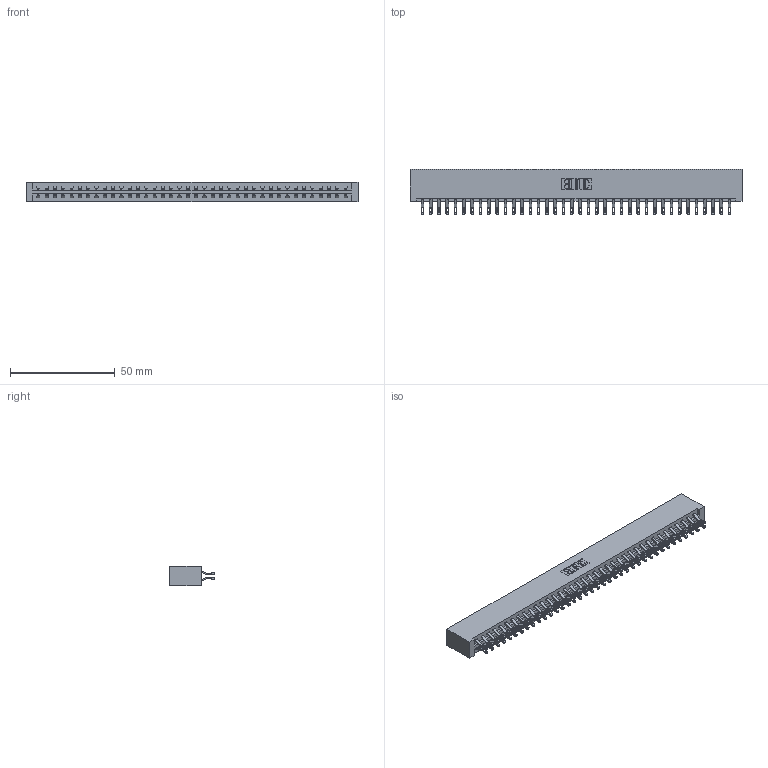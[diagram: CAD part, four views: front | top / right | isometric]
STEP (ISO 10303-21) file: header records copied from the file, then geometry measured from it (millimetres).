
FILE_DESCRIPTION (( 'STEP AP203' ), '1' );
FILE_NAME ('387-076-555-201.STEP', '2018-09-23T15:59:29', ( '' ), ( '' ), 'SwSTEP 2.0', 'SolidWorks 2016', '' );
FILE_SCHEMA (( 'CONFIG_CONTROL_DESIGN' ));
Length unit declared in the file: inch
Products named in the file (3): 337 Part_No Mounting Lugs; 345-292-001_555 Tail; 387-076-555-201
Assembly tree (77 placements, depth 2):
  387-076-555-201
    337 Part_No Mounting Lugs
    345-292-001_555 Tail  x76
Bounding box: 158.45 x 21.47 x 9.4 mm (x, y, z)
Volume: 17626.1 mm3; surface area: 20774.4 mm2
Topology: 77 solids, 77 shells, 4666 faces, 14651 edges, 9766 vertices
Faces by surface type: plane 2802, cylinder 1864
Entity records: 30029 total; most frequent: CARTESIAN_POINT 5096, ORIENTED_EDGE 5002, DIRECTION 4305, EDGE_CURVE 2501, VECTOR 2361, LINE 2361, VERTEX_POINT 1666, AXIS2_PLACEMENT_3D 972
